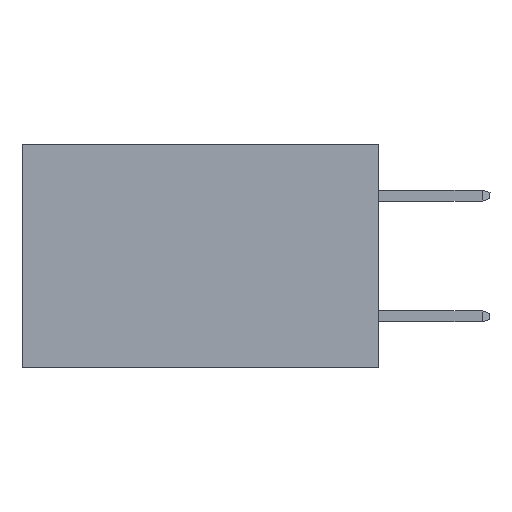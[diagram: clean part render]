
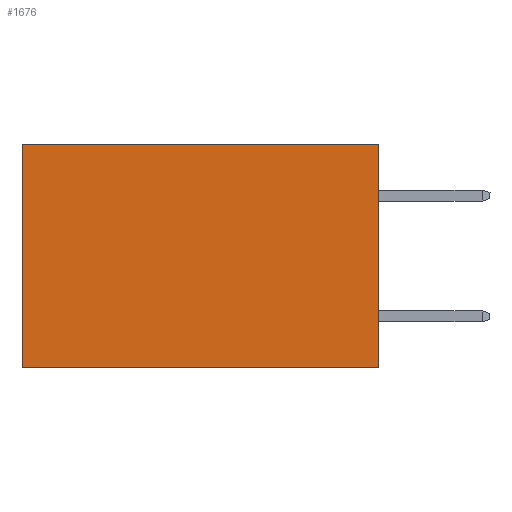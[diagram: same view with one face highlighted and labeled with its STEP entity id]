
A CAD part, left-side view. The second image highlights one B-rep face of the part: STEP entity #1676.
In plain terms, the highlighted planar face has unit normal (-1, 0, 0).
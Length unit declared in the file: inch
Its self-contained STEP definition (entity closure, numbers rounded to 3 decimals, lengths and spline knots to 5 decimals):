
#86 = AXIS2_PLACEMENT_3D ( 'NONE', #639, #2452, #2404 ) ;
#221 = LINE ( 'NONE', #3020, #10505 ) ;
#438 = DIRECTION ( 'NONE',  ( 0., 0., -1. ) ) ;
#639 = CARTESIAN_POINT ( 'NONE',  ( 0.277, 0., -0.37 ) ) ;
#1139 = VECTOR ( 'NONE', #2463, 39.37008 ) ;
#1297 = CARTESIAN_POINT ( 'NONE',  ( 0.277, 0.59, 0. ) ) ;
#1334 = EDGE_CURVE ( 'NONE', #3336, #9050, #221, .T. ) ;
#1337 = EDGE_CURVE ( 'NONE', #3924, #3336, #6843, .T. ) ;
#1676 = ADVANCED_FACE ( 'NONE', ( #7605 ), #8192, .F. ) ;
#1932 = CARTESIAN_POINT ( 'NONE',  ( 0.277, 0.59, -0.37 ) ) ;
#1942 = EDGE_CURVE ( 'NONE', #9182, #9050, #8165, .T. ) ;
#1964 = EDGE_CURVE ( 'NONE', #3924, #9182, #9696, .T. ) ;
#1987 = VECTOR ( 'NONE', #6860, 39.37008 ) ;
#2010 = ORIENTED_EDGE ( 'NONE', *, *, #1942, .F. ) ;
#2404 = DIRECTION ( 'NONE',  ( 0., 0., -1. ) ) ;
#2452 = DIRECTION ( 'NONE',  ( 1., 0., 0. ) ) ;
#2463 = DIRECTION ( 'NONE',  ( 0., 0., -1. ) ) ;
#2665 = CARTESIAN_POINT ( 'NONE',  ( 0.277, 0., 0. ) ) ;
#3020 = CARTESIAN_POINT ( 'NONE',  ( 0.277, 0.59, -0.37 ) ) ;
#3336 = VERTEX_POINT ( 'NONE', #1297 ) ;
#3566 = DIRECTION ( 'NONE',  ( 0., 1., 0. ) ) ;
#3924 = VERTEX_POINT ( 'NONE', #10094 ) ;
#4574 = ORIENTED_EDGE ( 'NONE', *, *, #1964, .F. ) ;
#5561 = EDGE_LOOP ( 'NONE', ( #10072, #2010, #4574, #6616 ) ) ;
#6234 = VECTOR ( 'NONE', #3566, 39.37008 ) ;
#6616 = ORIENTED_EDGE ( 'NONE', *, *, #1337, .T. ) ;
#6818 = CARTESIAN_POINT ( 'NONE',  ( 0.277, 0., -0.37 ) ) ;
#6843 = LINE ( 'NONE', #2665, #1987 ) ;
#6860 = DIRECTION ( 'NONE',  ( 0., 1., 0. ) ) ;
#7605 = FACE_OUTER_BOUND ( 'NONE', #5561, .T. ) ;
#8165 = LINE ( 'NONE', #6818, #6234 ) ;
#8192 = PLANE ( 'NONE',  #86 ) ;
#8294 = CARTESIAN_POINT ( 'NONE',  ( 0.277, 0., -0.37 ) ) ;
#8576 = CARTESIAN_POINT ( 'NONE',  ( 0.277, 0., -0.37 ) ) ;
#9050 = VERTEX_POINT ( 'NONE', #1932 ) ;
#9182 = VERTEX_POINT ( 'NONE', #8576 ) ;
#9696 = LINE ( 'NONE', #8294, #1139 ) ;
#10072 = ORIENTED_EDGE ( 'NONE', *, *, #1334, .T. ) ;
#10094 = CARTESIAN_POINT ( 'NONE',  ( 0.277, 0., 0. ) ) ;
#10505 = VECTOR ( 'NONE', #438, 39.37008 ) ;
